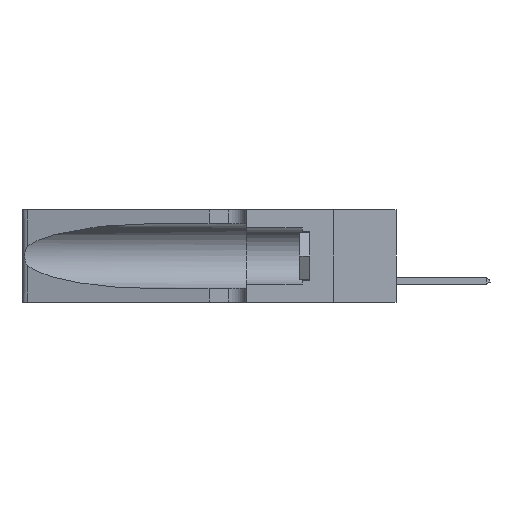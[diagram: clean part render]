
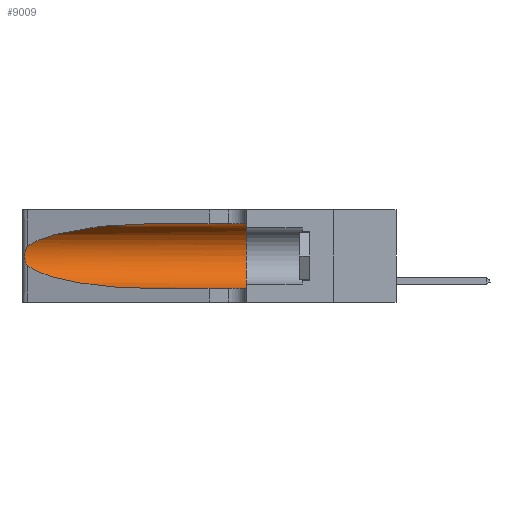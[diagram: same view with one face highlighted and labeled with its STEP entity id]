
A CAD part, left-side view. The second image highlights one B-rep face of the part: STEP entity #9009.
In plain terms, the highlighted cylindrical face has radius 3.308 mm (diameter 6.617 mm), a partial arc.
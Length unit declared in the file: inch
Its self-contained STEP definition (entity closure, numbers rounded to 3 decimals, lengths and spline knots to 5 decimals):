
#1091 = DIRECTION ( 'NONE',  ( 0., -1., 0. ) ) ;
#1396 = ORIENTED_EDGE ( 'NONE', *, *, #2605, .F. ) ;
#1423 = VERTEX_POINT ( 'NONE', #17119 ) ;
#1463 = CARTESIAN_POINT ( 'NONE',  ( 0.1305, 1.61858, 0.31525 ) ) ;
#1504 = CARTESIAN_POINT ( 'NONE',  ( 0.25555, 1.22994, 0.2215 ) ) ;
#1638 = CARTESIAN_POINT ( 'NONE',  ( 0.1305, 0.35, 0.05475 ) ) ;
#1930 = CARTESIAN_POINT ( 'NONE',  ( 0.25555, 1.22993, 0.14849 ) ) ;
#2605 = EDGE_CURVE ( 'NONE', #10580, #4699, #7773, .T. ) ;
#2618 =( BOUNDED_CURVE ( )  B_SPLINE_CURVE ( 3, ( #15872, #6033, #5120, #4825 ),
 .UNSPECIFIED., .F., .F. ) 
 B_SPLINE_CURVE_WITH_KNOTS ( ( 4, 4 ),
 ( 3.44316, 4.71239 ),
 .UNSPECIFIED. ) 
 CURVE ( )  GEOMETRIC_REPRESENTATION_ITEM ( )  RATIONAL_B_SPLINE_CURVE ( ( 1., 0.87, 0.87, 1. ) ) 
 REPRESENTATION_ITEM ( '' )  );
#2803 = CARTESIAN_POINT ( 'NONE',  ( 0.26075, 1.23896, 0.19203 ) ) ;
#3563 = CARTESIAN_POINT ( 'NONE',  ( 0.25856, 1.23593, 0.16098 ) ) ;
#4358 = CARTESIAN_POINT ( 'NONE',  ( 0.25787, 1.23484, 0.2124 ) ) ;
#4664 = CARTESIAN_POINT ( 'NONE',  ( 0.1305, 0.35, 0.185 ) ) ;
#4699 = VERTEX_POINT ( 'NONE', #1638 ) ;
#4825 = CARTESIAN_POINT ( 'NONE',  ( 0.1305, 0.72297, 0.05475 ) ) ;
#5120 = CARTESIAN_POINT ( 'NONE',  ( 0.18966, 0.96281, 0.05475 ) ) ;
#5209 = CARTESIAN_POINT ( 'NONE',  ( 0.25789, 1.23486, 0.15765 ) ) ;
#5673 = ORIENTED_EDGE ( 'NONE', *, *, #8554, .T. ) ;
#5767 = EDGE_CURVE ( 'NONE', #1423, #8494, #2618, .T. ) ;
#5831 = VERTEX_POINT ( 'NONE', #18465 ) ;
#6033 = CARTESIAN_POINT ( 'NONE',  ( 0.2373, 1.15595, 0.08982 ) ) ;
#6180 = VECTOR ( 'NONE', #6549, 39.37008 ) ;
#6549 = DIRECTION ( 'NONE',  ( 0., -1., 0. ) ) ;
#7634 = DIRECTION ( 'NONE',  ( 0., -1., 0. ) ) ;
#7738 = CARTESIAN_POINT ( 'NONE',  ( 0.26018, 1.23835, 0.19895 ) ) ;
#7773 = CIRCLE ( 'NONE', #8303, 0.13025 ) ;
#8035 = CARTESIAN_POINT ( 'NONE',  ( 0.26075, 1.23896, 0.178 ) ) ;
#8303 = AXIS2_PLACEMENT_3D ( 'NONE', #4664, #10923, #14050 ) ;
#8456 = VECTOR ( 'NONE', #7634, 39.37008 ) ;
#8493 = CARTESIAN_POINT ( 'NONE',  ( 0.2373, 1.15595, 0.28018 ) ) ;
#8494 = VERTEX_POINT ( 'NONE', #14411 ) ;
#8554 = EDGE_CURVE ( 'NONE', #8494, #4699, #14463, .T. ) ;
#8901 = DIRECTION ( 'NONE',  ( 0., 0., -1. ) ) ;
#9009 = ADVANCED_FACE ( 'NONE', ( #14468 ), #18620, .F. ) ;
#10102 = ORIENTED_EDGE ( 'NONE', *, *, #5767, .T. ) ;
#10311 = EDGE_CURVE ( 'NONE', #18082, #1423, #18201, .T. ) ;
#10580 = VERTEX_POINT ( 'NONE', #16501 ) ;
#10824 = CARTESIAN_POINT ( 'NONE',  ( 0.25487, 1.22718, 0.22369 ) ) ;
#10923 = DIRECTION ( 'NONE',  ( 0., 1., 0. ) ) ;
#11261 = CARTESIAN_POINT ( 'NONE',  ( 0.26017, 1.23833, 0.17102 ) ) ;
#11649 = CARTESIAN_POINT ( 'NONE',  ( 0.25487, 1.22718, 0.22369 ) ) ;
#11744 = ORIENTED_EDGE ( 'NONE', *, *, #14262, .T. ) ;
#11826 = ORIENTED_EDGE ( 'NONE', *, *, #12601, .F. ) ;
#12053 = AXIS2_PLACEMENT_3D ( 'NONE', #19756, #1091, #8901 ) ;
#12216 = EDGE_LOOP ( 'NONE', ( #11744, #16291, #10102, #5673, #1396, #11826 ) ) ;
#12601 = EDGE_CURVE ( 'NONE', #5831, #10580, #19186, .T. ) ;
#14000 = CARTESIAN_POINT ( 'NONE',  ( 0.1305, 1.61858, 0.05475 ) ) ;
#14050 = DIRECTION ( 'NONE',  ( 0., 0., 1. ) ) ;
#14238 = CARTESIAN_POINT ( 'NONE',  ( 0.25487, 1.22718, 0.14631 ) ) ;
#14262 = EDGE_CURVE ( 'NONE', #5831, #18082, #15213, .T. ) ;
#14411 = CARTESIAN_POINT ( 'NONE',  ( 0.1305, 0.72297, 0.05475 ) ) ;
#14463 = LINE ( 'NONE', #14000, #6180 ) ;
#14468 = FACE_OUTER_BOUND ( 'NONE', #12216, .T. ) ;
#15213 =( BOUNDED_CURVE ( )  B_SPLINE_CURVE ( 3, ( #16213, #19125, #8493, #11649 ),
 .UNSPECIFIED., .F., .F. ) 
 B_SPLINE_CURVE_WITH_KNOTS ( ( 4, 4 ),
 ( 1.5708, 2.84003 ),
 .UNSPECIFIED. ) 
 CURVE ( )  GEOMETRIC_REPRESENTATION_ITEM ( )  RATIONAL_B_SPLINE_CURVE ( ( 1., 0.87, 0.87, 1. ) ) 
 REPRESENTATION_ITEM ( '' )  );
#15872 = CARTESIAN_POINT ( 'NONE',  ( 0.25487, 1.22718, 0.14631 ) ) ;
#16106 = CARTESIAN_POINT ( 'NONE',  ( 0.25639, 1.23186, 0.15144 ) ) ;
#16213 = CARTESIAN_POINT ( 'NONE',  ( 0.1305, 0.72297, 0.31525 ) ) ;
#16291 = ORIENTED_EDGE ( 'NONE', *, *, #10311, .T. ) ;
#16501 = CARTESIAN_POINT ( 'NONE',  ( 0.1305, 0.35, 0.31525 ) ) ;
#16572 = CARTESIAN_POINT ( 'NONE',  ( 0.25487, 1.22718, 0.22369 ) ) ;
#16828 = CARTESIAN_POINT ( 'NONE',  ( 0.25854, 1.2359, 0.20912 ) ) ;
#17085 = CARTESIAN_POINT ( 'NONE',  ( 0.25639, 1.23184, 0.21858 ) ) ;
#17119 = CARTESIAN_POINT ( 'NONE',  ( 0.25487, 1.22718, 0.14631 ) ) ;
#18082 = VERTEX_POINT ( 'NONE', #16572 ) ;
#18201 = B_SPLINE_CURVE_WITH_KNOTS ( 'NONE', 3,
 ( #10824, #1504, #17085, #4358, #16828, #7738, #2803, #8035, #11261, #3563, #5209, #16106, #1930, #14238 ),
 .UNSPECIFIED., .F., .F.,
 ( 4, 2, 2, 2, 2, 2, 4 ),
 ( 0., 0.00027, 0.00053, 0.00107, 0.0016, 0.00187, 0.00214 ),
 .UNSPECIFIED. ) ;
#18465 = CARTESIAN_POINT ( 'NONE',  ( 0.1305, 0.72297, 0.31525 ) ) ;
#18620 = CYLINDRICAL_SURFACE ( 'NONE', #12053, 0.13025 ) ;
#19125 = CARTESIAN_POINT ( 'NONE',  ( 0.18966, 0.96281, 0.31525 ) ) ;
#19186 = LINE ( 'NONE', #1463, #8456 ) ;
#19756 = CARTESIAN_POINT ( 'NONE',  ( 0.1305, 1.61858, 0.185 ) ) ;
